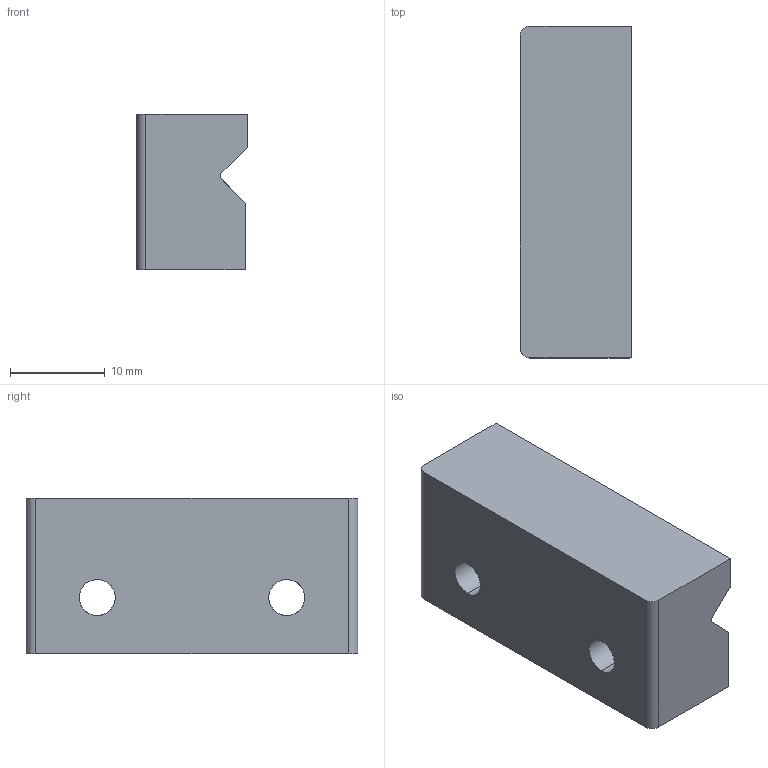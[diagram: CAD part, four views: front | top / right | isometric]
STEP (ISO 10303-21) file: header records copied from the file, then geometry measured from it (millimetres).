
FILE_DESCRIPTION (( 'STEP AP203' ), '1' );
FILE_NAME ('rail keeper.STEP', '2020-10-26T18:38:23', ( '' ), ( '' ), 'SwSTEP 2.0', 'SolidWorks 2019', '' );
FILE_SCHEMA (( 'CONFIG_CONTROL_DESIGN' ));
Length unit declared in the file: millimetre
Products named in the file (1): rail keeper
Bounding box: 11.73 x 35 x 16.4 mm (x, y, z)
Volume: 6073.4 mm3; surface area: 2607.8 mm2
Topology: 1 solids, 1 shells, 16 faces, 48 edges, 32 vertices
Faces by surface type: plane 9, cylinder 7
Entity records: 631 total; most frequent: CARTESIAN_POINT 109, ORIENTED_EDGE 96, DIRECTION 92, EDGE_CURVE 48, VERTEX_POINT 32, AXIS2_PLACEMENT_3D 31, VECTOR 30, LINE 30
